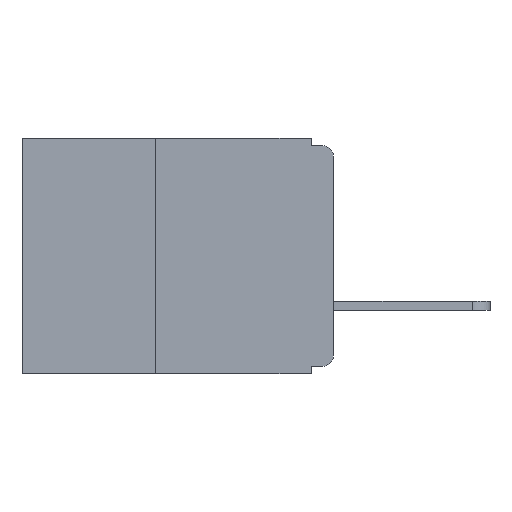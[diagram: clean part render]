
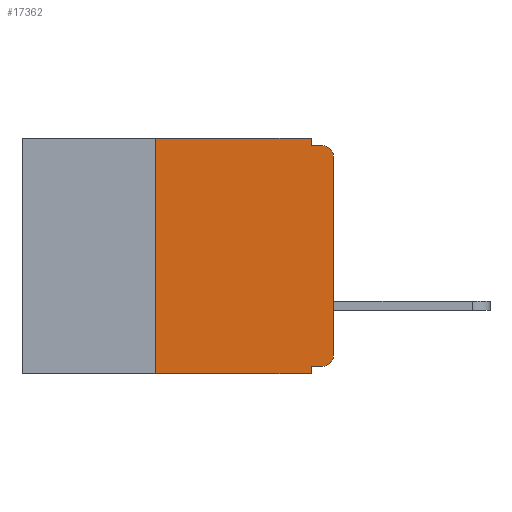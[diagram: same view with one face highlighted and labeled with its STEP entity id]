
A CAD part, left-side view. The second image highlights one B-rep face of the part: STEP entity #17362.
In plain terms, the highlighted planar face has unit normal (-1, 0, 0).
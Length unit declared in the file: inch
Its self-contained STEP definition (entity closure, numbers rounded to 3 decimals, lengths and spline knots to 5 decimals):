
#50 = DIRECTION ( 'NONE',  ( -1., 0., 0. ) ) ;
#433 = CARTESIAN_POINT ( 'NONE',  ( 0., 0., -0.32 ) ) ;
#1725 = VERTEX_POINT ( 'NONE', #14657 ) ;
#1871 = VERTEX_POINT ( 'NONE', #21492 ) ;
#2180 = EDGE_LOOP ( 'NONE', ( #6545, #7058, #17151, #11486, #17660, #23147, #11269, #13433, #11199, #20711 ) ) ;
#2290 = EDGE_CURVE ( 'NONE', #16382, #4248, #17787, .T. ) ;
#2748 = DIRECTION ( 'NONE',  ( 0., -1., 0. ) ) ;
#2875 = EDGE_CURVE ( 'NONE', #15620, #1871, #24620, .T. ) ;
#3020 = CARTESIAN_POINT ( 'NONE',  ( 0., 0.437, 0. ) ) ;
#3047 = CIRCLE ( 'NONE', #15481, 0.015 ) ;
#3127 = CARTESIAN_POINT ( 'NONE',  ( 0., 0.25, 0. ) ) ;
#4152 = LINE ( 'NONE', #3020, #15222 ) ;
#4244 = PLANE ( 'NONE',  #23294 ) ;
#4248 = VERTEX_POINT ( 'NONE', #11251 ) ;
#4534 = EDGE_CURVE ( 'NONE', #22038, #1725, #4152, .T. ) ;
#4561 = LINE ( 'NONE', #26029, #27984 ) ;
#5100 = CIRCLE ( 'NONE', #17639, 0.015 ) ;
#6411 = CARTESIAN_POINT ( 'NONE',  ( 0., 0.015, -0.305 ) ) ;
#6510 = LINE ( 'NONE', #23190, #23445 ) ;
#6545 = ORIENTED_EDGE ( 'NONE', *, *, #2875, .T. ) ;
#6559 = CARTESIAN_POINT ( 'NONE',  ( 0., 0.437, -0.33 ) ) ;
#6586 = VERTEX_POINT ( 'NONE', #24326 ) ;
#6615 = DIRECTION ( 'NONE',  ( 0., 0., -1. ) ) ;
#6991 = LINE ( 'NONE', #16688, #23215 ) ;
#7058 = ORIENTED_EDGE ( 'NONE', *, *, #18841, .T. ) ;
#7273 = DIRECTION ( 'NONE',  ( 0., -1., 0. ) ) ;
#7377 = VERTEX_POINT ( 'NONE', #25398 ) ;
#8245 = EDGE_CURVE ( 'NONE', #16382, #22038, #4561, .T. ) ;
#8674 = DIRECTION ( 'NONE',  ( 0., 0., -1. ) ) ;
#10616 = DIRECTION ( 'NONE',  ( 0., 0., 1. ) ) ;
#11011 = CARTESIAN_POINT ( 'NONE',  ( 0., 0.015, -0.01 ) ) ;
#11012 = CARTESIAN_POINT ( 'NONE',  ( 0., 0., 0. ) ) ;
#11037 = CARTESIAN_POINT ( 'NONE',  ( 0., 0.437, 0. ) ) ;
#11181 = DIRECTION ( 'NONE',  ( 0., 0., 1. ) ) ;
#11199 = ORIENTED_EDGE ( 'NONE', *, *, #24723, .F. ) ;
#11201 = EDGE_CURVE ( 'NONE', #1725, #7377, #23080, .T. ) ;
#11251 = CARTESIAN_POINT ( 'NONE',  ( 0., 0.031, -0.33 ) ) ;
#11269 = ORIENTED_EDGE ( 'NONE', *, *, #2290, .T. ) ;
#11486 = ORIENTED_EDGE ( 'NONE', *, *, #11201, .F. ) ;
#12140 = CARTESIAN_POINT ( 'NONE',  ( 0., 0.031, -0.32 ) ) ;
#12409 = VERTEX_POINT ( 'NONE', #12140 ) ;
#13234 = DIRECTION ( 'NONE',  ( 0., 0., -1. ) ) ;
#13307 = CARTESIAN_POINT ( 'NONE',  ( 0., 0.015, -0.025 ) ) ;
#13433 = ORIENTED_EDGE ( 'NONE', *, *, #27926, .F. ) ;
#14358 = EDGE_CURVE ( 'NONE', #6586, #15620, #3047, .T. ) ;
#14657 = CARTESIAN_POINT ( 'NONE',  ( 0., 0.031, 0. ) ) ;
#15222 = VECTOR ( 'NONE', #2748, 39.37008 ) ;
#15284 = EDGE_CURVE ( 'NONE', #7377, #18820, #6510, .T. ) ;
#15481 = AXIS2_PLACEMENT_3D ( 'NONE', #6411, #21898, #8674 ) ;
#15542 = DIRECTION ( 'NONE',  ( 0., 0., -1. ) ) ;
#15558 = CARTESIAN_POINT ( 'NONE',  ( 0., 0., -0.305 ) ) ;
#15620 = VERTEX_POINT ( 'NONE', #15558 ) ;
#15927 = DIRECTION ( 'NONE',  ( 0., 1., 0. ) ) ;
#16382 = VERTEX_POINT ( 'NONE', #27135 ) ;
#16688 = CARTESIAN_POINT ( 'NONE',  ( 0., 0.031, -0.33 ) ) ;
#17077 = VECTOR ( 'NONE', #7273, 39.37008 ) ;
#17151 = ORIENTED_EDGE ( 'NONE', *, *, #15284, .F. ) ;
#17362 = ADVANCED_FACE ( 'NONE', ( #19550 ), #4244, .F. ) ;
#17639 = AXIS2_PLACEMENT_3D ( 'NONE', #13307, #50, #15542 ) ;
#17660 = ORIENTED_EDGE ( 'NONE', *, *, #4534, .F. ) ;
#17674 = CARTESIAN_POINT ( 'NONE',  ( 0., 0.031, 0. ) ) ;
#17787 = LINE ( 'NONE', #6559, #17077 ) ;
#18635 = VECTOR ( 'NONE', #15927, 39.37008 ) ;
#18779 = VECTOR ( 'NONE', #11181, 39.37008 ) ;
#18820 = VERTEX_POINT ( 'NONE', #11011 ) ;
#18841 = EDGE_CURVE ( 'NONE', #1871, #18820, #5100, .T. ) ;
#18941 = DIRECTION ( 'NONE',  ( 0., 0., -1. ) ) ;
#19550 = FACE_OUTER_BOUND ( 'NONE', #2180, .T. ) ;
#20711 = ORIENTED_EDGE ( 'NONE', *, *, #14358, .T. ) ;
#21492 = CARTESIAN_POINT ( 'NONE',  ( 0., 0., -0.025 ) ) ;
#21898 = DIRECTION ( 'NONE',  ( -1., 0., 0. ) ) ;
#22038 = VERTEX_POINT ( 'NONE', #3127 ) ;
#22416 = VECTOR ( 'NONE', #6615, 39.37008 ) ;
#23080 = LINE ( 'NONE', #17674, #22416 ) ;
#23147 = ORIENTED_EDGE ( 'NONE', *, *, #8245, .F. ) ;
#23190 = CARTESIAN_POINT ( 'NONE',  ( 0., 0., -0.01 ) ) ;
#23215 = VECTOR ( 'NONE', #18941, 39.37008 ) ;
#23294 = AXIS2_PLACEMENT_3D ( 'NONE', #11037, #26460, #13234 ) ;
#23445 = VECTOR ( 'NONE', #25400, 39.37008 ) ;
#24326 = CARTESIAN_POINT ( 'NONE',  ( 0., 0.015, -0.32 ) ) ;
#24466 = LINE ( 'NONE', #433, #18635 ) ;
#24620 = LINE ( 'NONE', #11012, #18779 ) ;
#24723 = EDGE_CURVE ( 'NONE', #6586, #12409, #24466, .T. ) ;
#25398 = CARTESIAN_POINT ( 'NONE',  ( 0., 0.031, -0.01 ) ) ;
#25400 = DIRECTION ( 'NONE',  ( 0., -1., 0. ) ) ;
#26029 = CARTESIAN_POINT ( 'NONE',  ( 0., 0.25, -0.33 ) ) ;
#26460 = DIRECTION ( 'NONE',  ( 1., 0., 0. ) ) ;
#27135 = CARTESIAN_POINT ( 'NONE',  ( 0., 0.25, -0.33 ) ) ;
#27926 = EDGE_CURVE ( 'NONE', #12409, #4248, #6991, .T. ) ;
#27984 = VECTOR ( 'NONE', #10616, 39.37008 ) ;
